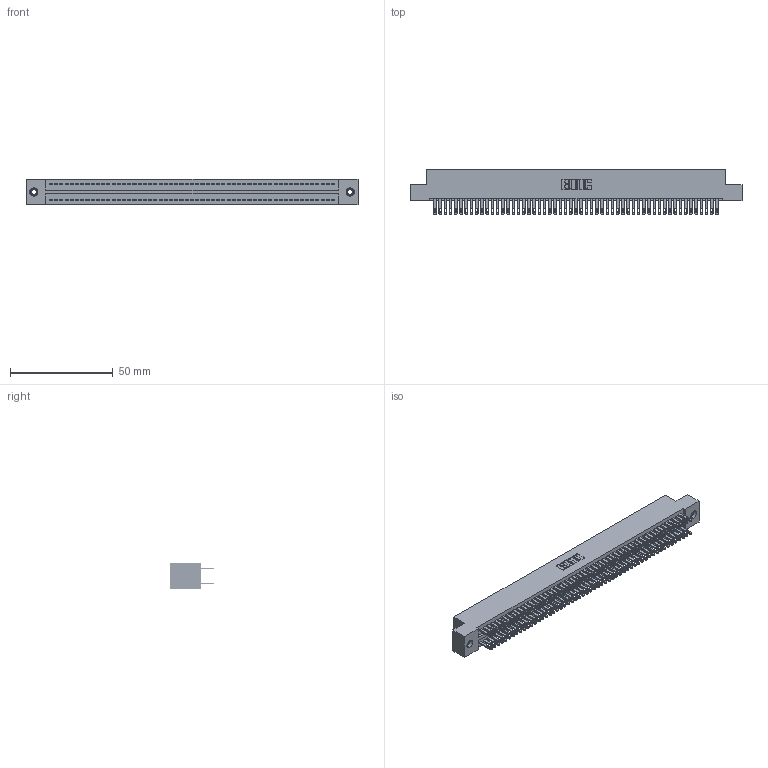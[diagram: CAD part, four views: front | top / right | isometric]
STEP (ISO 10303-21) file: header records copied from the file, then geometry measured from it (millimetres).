
FILE_DESCRIPTION (( 'STEP AP203' ), '1' );
FILE_NAME ('325-110-500-207.STEP', '2020-02-25T07:35:13', ( '' ), ( '' ), 'SwSTEP 2.0', 'SolidWorks 2016', '' );
FILE_SCHEMA (( 'CONFIG_CONTROL_DESIGN' ));
Length unit declared in the file: inch
Products named in the file (4): 325-292-001_325-293-100; 325-110-500-207; 345-250-001_345-250-005-103; 325 Part_TI
Assembly tree (113 placements, depth 2):
  325-110-500-207
    325 Part_TI
    325-292-001_325-293-100  x110
    345-250-001_345-250-005-103  x2
Bounding box: 161.42 x 21.84 x 12.45 mm (x, y, z)
Volume: 21277.5 mm3; surface area: 27238.3 mm2
Topology: 113 solids, 113 shells, 5454 faces, 16617 edges, 11070 vertices
Faces by surface type: plane 3402, cylinder 2036, cone 12, torus 4
Entity records: 34818 total; most frequent: CARTESIAN_POINT 5737, ORIENTED_EDGE 5666, DIRECTION 4911, EDGE_CURVE 2833, VECTOR 2681, LINE 2681, VERTEX_POINT 1884, AXIS2_PLACEMENT_3D 1115
